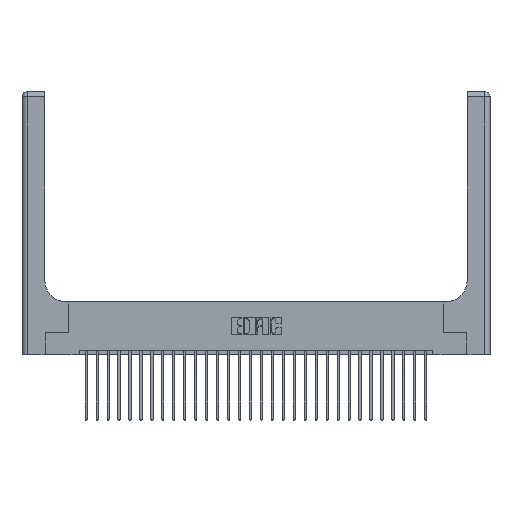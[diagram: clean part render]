
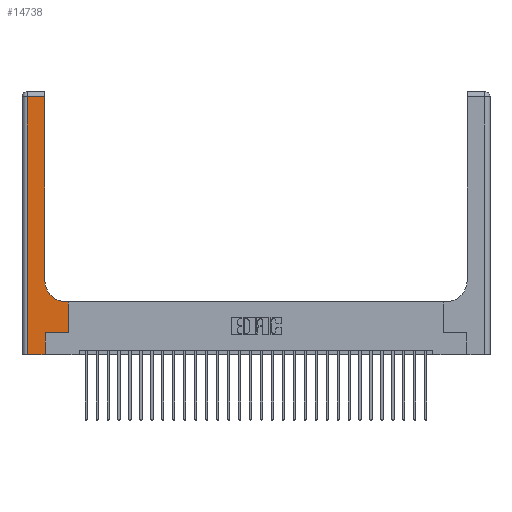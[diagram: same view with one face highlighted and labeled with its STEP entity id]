
A CAD part, top view. The second image highlights one B-rep face of the part: STEP entity #14738.
In plain terms, the highlighted planar face has unit normal (0, 0, 1).
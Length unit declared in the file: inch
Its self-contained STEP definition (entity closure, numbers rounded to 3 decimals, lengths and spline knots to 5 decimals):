
#692 = LINE ( 'NONE', #2811, #5401 ) ;
#770 = VECTOR ( 'NONE', #3520, 39.37008 ) ;
#1043 = EDGE_CURVE ( 'NONE', #11647, #24905, #3326, .T. ) ;
#1111 = EDGE_CURVE ( 'NONE', #18575, #11056, #15561, .T. ) ;
#1195 = VECTOR ( 'NONE', #27023, 39.37008 ) ;
#1669 = DIRECTION ( 'NONE',  ( -1., 0., 0. ) ) ;
#2158 = CARTESIAN_POINT ( 'NONE',  ( 0.26, 0.85, 0.37 ) ) ;
#2479 = VERTEX_POINT ( 'NONE', #23298 ) ;
#2574 = VERTEX_POINT ( 'NONE', #22019 ) ;
#2811 = CARTESIAN_POINT ( 'NONE',  ( 0.265, 0., 0.37 ) ) ;
#2907 = DIRECTION ( 'NONE',  ( 0., 0., -1. ) ) ;
#2913 = VECTOR ( 'NONE', #11918, 39.37008 ) ;
#3077 = VECTOR ( 'NONE', #11905, 39.37008 ) ;
#3216 = VECTOR ( 'NONE', #18605, 39.37008 ) ;
#3326 = LINE ( 'NONE', #22784, #26371 ) ;
#3520 = DIRECTION ( 'NONE',  ( -1., 0., 0. ) ) ;
#4298 = EDGE_CURVE ( 'NONE', #6511, #18575, #13677, .T. ) ;
#4467 = EDGE_CURVE ( 'NONE', #2479, #6511, #20996, .T. ) ;
#4784 = ORIENTED_EDGE ( 'NONE', *, *, #1043, .T. ) ;
#5401 = VECTOR ( 'NONE', #11282, 39.37008 ) ;
#5426 = CARTESIAN_POINT ( 'NONE',  ( 0., 0., 0.37 ) ) ;
#5795 = VERTEX_POINT ( 'NONE', #25513 ) ;
#6196 = LINE ( 'NONE', #14650, #3216 ) ;
#6511 = VERTEX_POINT ( 'NONE', #10879 ) ;
#6652 = CARTESIAN_POINT ( 'NONE',  ( 0.26, 2.94, 0.37 ) ) ;
#7364 = EDGE_LOOP ( 'NONE', ( #8870, #16006, #4784, #20870, #18532, #27206, #15461, #13913, #10256 ) ) ;
#7432 = CARTESIAN_POINT ( 'NONE',  ( 0.51, 0.85, 0.37 ) ) ;
#8027 = PLANE ( 'NONE',  #9359 ) ;
#8870 = ORIENTED_EDGE ( 'NONE', *, *, #10741, .T. ) ;
#9260 = DIRECTION ( 'NONE',  ( 0., -1., 0. ) ) ;
#9359 = AXIS2_PLACEMENT_3D ( 'NONE', #16645, #25227, #1669 ) ;
#10256 = ORIENTED_EDGE ( 'NONE', *, *, #1111, .T. ) ;
#10741 = EDGE_CURVE ( 'NONE', #11056, #12734, #24044, .T. ) ;
#10879 = CARTESIAN_POINT ( 'NONE',  ( 0.528, 0.6, 0.37 ) ) ;
#11056 = VERTEX_POINT ( 'NONE', #2158 ) ;
#11282 = DIRECTION ( 'NONE',  ( 0., 1., 0. ) ) ;
#11647 = VERTEX_POINT ( 'NONE', #20447 ) ;
#11905 = DIRECTION ( 'NONE',  ( 1., 0., 0. ) ) ;
#11918 = DIRECTION ( 'NONE',  ( 0., 1., 0. ) ) ;
#12734 = VERTEX_POINT ( 'NONE', #6652 ) ;
#13677 = LINE ( 'NONE', #26663, #770 ) ;
#13791 = EDGE_CURVE ( 'NONE', #2574, #2479, #23048, .T. ) ;
#13913 = ORIENTED_EDGE ( 'NONE', *, *, #4298, .T. ) ;
#14038 = CARTESIAN_POINT ( 'NONE',  ( 0.26, 3., 0.37 ) ) ;
#14650 = CARTESIAN_POINT ( 'NONE',  ( 0., 2.94, 0.37 ) ) ;
#14738 = ADVANCED_FACE ( 'NONE', ( #25084 ), #8027, .F. ) ;
#15461 = ORIENTED_EDGE ( 'NONE', *, *, #4467, .T. ) ;
#15561 = CIRCLE ( 'NONE', #20070, 0.25 ) ;
#16006 = ORIENTED_EDGE ( 'NONE', *, *, #27869, .T. ) ;
#16645 = CARTESIAN_POINT ( 'NONE',  ( 0., 3., 0.37 ) ) ;
#18296 = DIRECTION ( 'NONE',  ( 1., 0., 0. ) ) ;
#18418 = CARTESIAN_POINT ( 'NONE',  ( 0.265, 0.25, 0.37 ) ) ;
#18532 = ORIENTED_EDGE ( 'NONE', *, *, #23951, .T. ) ;
#18575 = VERTEX_POINT ( 'NONE', #21733 ) ;
#18605 = DIRECTION ( 'NONE',  ( -1., 0., 0. ) ) ;
#20070 = AXIS2_PLACEMENT_3D ( 'NONE', #7432, #2907, #18296 ) ;
#20447 = CARTESIAN_POINT ( 'NONE',  ( 0.06, 2.94, 0.37 ) ) ;
#20644 = LINE ( 'NONE', #5426, #3077 ) ;
#20870 = ORIENTED_EDGE ( 'NONE', *, *, #22693, .T. ) ;
#20996 = LINE ( 'NONE', #23241, #26862 ) ;
#21030 = CARTESIAN_POINT ( 'NONE',  ( 0.06, 0., 0.37 ) ) ;
#21733 = CARTESIAN_POINT ( 'NONE',  ( 0.51, 0.6, 0.37 ) ) ;
#22019 = CARTESIAN_POINT ( 'NONE',  ( 0.265, 0.25, 0.37 ) ) ;
#22693 = EDGE_CURVE ( 'NONE', #24905, #5795, #20644, .T. ) ;
#22784 = CARTESIAN_POINT ( 'NONE',  ( 0.06, 3., 0.37 ) ) ;
#23048 = LINE ( 'NONE', #18418, #1195 ) ;
#23241 = CARTESIAN_POINT ( 'NONE',  ( 0.528, 0.25, 0.37 ) ) ;
#23298 = CARTESIAN_POINT ( 'NONE',  ( 0.528, 0.25, 0.37 ) ) ;
#23951 = EDGE_CURVE ( 'NONE', #5795, #2574, #692, .T. ) ;
#24044 = LINE ( 'NONE', #14038, #2913 ) ;
#24905 = VERTEX_POINT ( 'NONE', #21030 ) ;
#25084 = FACE_OUTER_BOUND ( 'NONE', #7364, .T. ) ;
#25227 = DIRECTION ( 'NONE',  ( 0., 0., -1. ) ) ;
#25513 = CARTESIAN_POINT ( 'NONE',  ( 0.265, 0., 0.37 ) ) ;
#26371 = VECTOR ( 'NONE', #9260, 39.37008 ) ;
#26663 = CARTESIAN_POINT ( 'NONE',  ( 0.26, 0.6, 0.37 ) ) ;
#26862 = VECTOR ( 'NONE', #27766, 39.37008 ) ;
#27023 = DIRECTION ( 'NONE',  ( 1., 0., 0. ) ) ;
#27206 = ORIENTED_EDGE ( 'NONE', *, *, #13791, .T. ) ;
#27766 = DIRECTION ( 'NONE',  ( 0., 1., 0. ) ) ;
#27869 = EDGE_CURVE ( 'NONE', #12734, #11647, #6196, .T. ) ;
